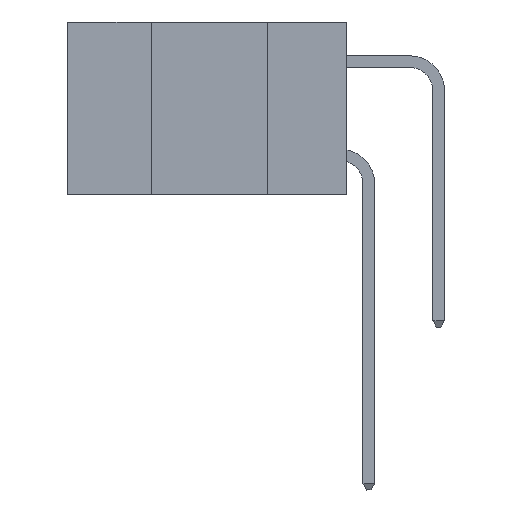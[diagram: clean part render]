
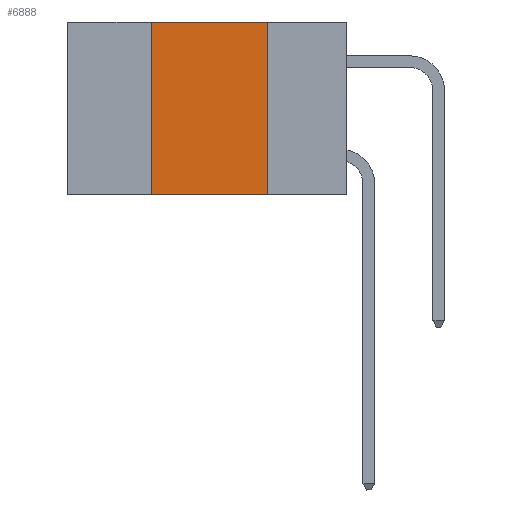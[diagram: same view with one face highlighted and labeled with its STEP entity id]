
A CAD part, left-side view. The second image highlights one B-rep face of the part: STEP entity #6888.
In plain terms, the highlighted planar face has unit normal (-1, 0, 0).
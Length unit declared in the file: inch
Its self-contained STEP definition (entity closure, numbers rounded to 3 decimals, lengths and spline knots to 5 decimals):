
#352 = CARTESIAN_POINT ( 'NONE',  ( 0., 0.42, 0. ) ) ;
#418 = EDGE_CURVE ( 'NONE', #30177, #28177, #15868, .T. ) ;
#736 = LINE ( 'NONE', #17988, #13708 ) ;
#1512 = EDGE_CURVE ( 'NONE', #26268, #27317, #736, .T. ) ;
#2517 = VECTOR ( 'NONE', #20500, 39.37008 ) ;
#2908 = LINE ( 'NONE', #20732, #2517 ) ;
#4074 = PLANE ( 'NONE',  #17078 ) ;
#4196 = DIRECTION ( 'NONE',  ( 0., 0., 1. ) ) ;
#6888 = ADVANCED_FACE ( 'NONE', ( #13369 ), #4074, .F. ) ;
#8142 = CARTESIAN_POINT ( 'NONE',  ( 0., 0.42, -0.37 ) ) ;
#10224 = CARTESIAN_POINT ( 'NONE',  ( 0., 0.17, -0.37 ) ) ;
#10901 = EDGE_LOOP ( 'NONE', ( #11893, #15074, #12205, #27467 ) ) ;
#11758 = CARTESIAN_POINT ( 'NONE',  ( 0., 0.6, 0. ) ) ;
#11893 = ORIENTED_EDGE ( 'NONE', *, *, #418, .F. ) ;
#12205 = ORIENTED_EDGE ( 'NONE', *, *, #1512, .F. ) ;
#13369 = FACE_OUTER_BOUND ( 'NONE', #10901, .T. ) ;
#13572 = VECTOR ( 'NONE', #28549, 39.37008 ) ;
#13708 = VECTOR ( 'NONE', #4196, 39.37008 ) ;
#15074 = ORIENTED_EDGE ( 'NONE', *, *, #27380, .F. ) ;
#15868 = LINE ( 'NONE', #21260, #33045 ) ;
#17078 = AXIS2_PLACEMENT_3D ( 'NONE', #11758, #27914, #33424 ) ;
#17988 = CARTESIAN_POINT ( 'NONE',  ( 0., 0.42, 0. ) ) ;
#18789 = EDGE_CURVE ( 'NONE', #26268, #28177, #2908, .T. ) ;
#20500 = DIRECTION ( 'NONE',  ( 0., -1., 0. ) ) ;
#20732 = CARTESIAN_POINT ( 'NONE',  ( 0., 0.6, -0.37 ) ) ;
#21260 = CARTESIAN_POINT ( 'NONE',  ( 0., 0.17, 0. ) ) ;
#24399 = LINE ( 'NONE', #28901, #13572 ) ;
#25462 = CARTESIAN_POINT ( 'NONE',  ( 0., 0.17, 0. ) ) ;
#26268 = VERTEX_POINT ( 'NONE', #8142 ) ;
#27317 = VERTEX_POINT ( 'NONE', #352 ) ;
#27380 = EDGE_CURVE ( 'NONE', #27317, #30177, #24399, .T. ) ;
#27467 = ORIENTED_EDGE ( 'NONE', *, *, #18789, .T. ) ;
#27914 = DIRECTION ( 'NONE',  ( 1., 0., 0. ) ) ;
#28177 = VERTEX_POINT ( 'NONE', #10224 ) ;
#28549 = DIRECTION ( 'NONE',  ( 0., -1., 0. ) ) ;
#28901 = CARTESIAN_POINT ( 'NONE',  ( 0., 0.6, 0. ) ) ;
#30177 = VERTEX_POINT ( 'NONE', #25462 ) ;
#33045 = VECTOR ( 'NONE', #34507, 39.37008 ) ;
#33424 = DIRECTION ( 'NONE',  ( 0., 0., -1. ) ) ;
#34507 = DIRECTION ( 'NONE',  ( 0., 0., -1. ) ) ;
